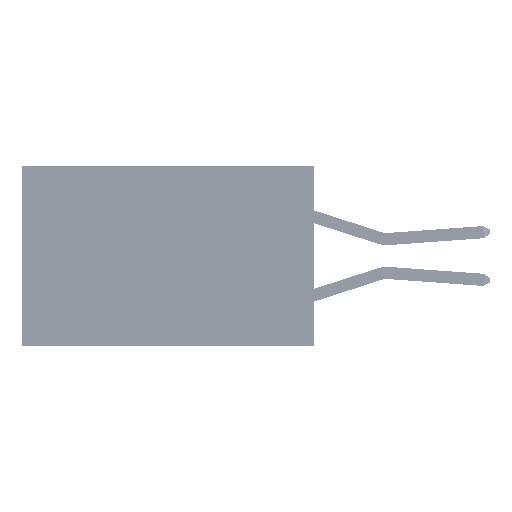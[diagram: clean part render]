
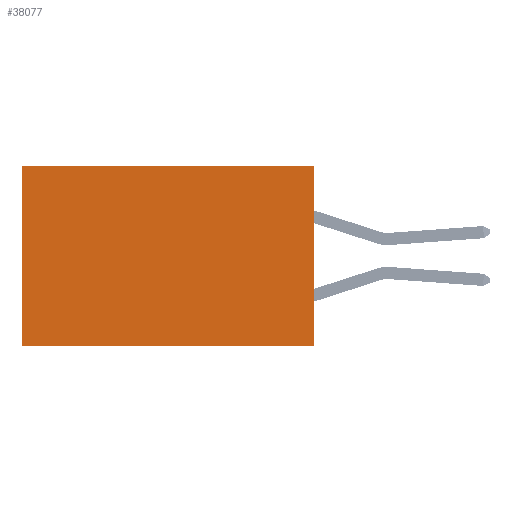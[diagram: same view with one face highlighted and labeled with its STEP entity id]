
A CAD part, left-side view. The second image highlights one B-rep face of the part: STEP entity #38077.
In plain terms, the highlighted planar face has unit normal (-1, 0, 0).
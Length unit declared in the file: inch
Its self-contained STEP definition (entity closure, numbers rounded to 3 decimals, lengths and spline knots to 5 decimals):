
#411 = VERTEX_POINT ( 'NONE', #23533 ) ;
#2952 = ORIENTED_EDGE ( 'NONE', *, *, #38654, .F. ) ;
#3434 = FACE_OUTER_BOUND ( 'NONE', #4018, .T. ) ;
#3687 = ORIENTED_EDGE ( 'NONE', *, *, #8347, .T. ) ;
#4018 = EDGE_LOOP ( 'NONE', ( #3687, #27992, #2952, #43859 ) ) ;
#5990 = VECTOR ( 'NONE', #41328, 39.37008 ) ;
#7865 = EDGE_CURVE ( 'NONE', #411, #35068, #50185, .T. ) ;
#8347 = EDGE_CURVE ( 'NONE', #35068, #29276, #51394, .T. ) ;
#9058 = VECTOR ( 'NONE', #41495, 39.37008 ) ;
#15047 = DIRECTION ( 'NONE',  ( 0., 0., -1. ) ) ;
#17683 = CARTESIAN_POINT ( 'NONE',  ( 0.2875, 0., 0. ) ) ;
#18601 = LINE ( 'NONE', #17683, #9058 ) ;
#19159 = PLANE ( 'NONE',  #27684 ) ;
#20217 = LINE ( 'NONE', #48362, #41045 ) ;
#22515 = CARTESIAN_POINT ( 'NONE',  ( 0.2875, 0., 0. ) ) ;
#23533 = CARTESIAN_POINT ( 'NONE',  ( 0.2875, 0., 0. ) ) ;
#25495 = EDGE_CURVE ( 'NONE', #47057, #29276, #20217, .T. ) ;
#26878 = DIRECTION ( 'NONE',  ( 0., 0., -1. ) ) ;
#27684 = AXIS2_PLACEMENT_3D ( 'NONE', #22515, #30951, #26878 ) ;
#27992 = ORIENTED_EDGE ( 'NONE', *, *, #25495, .F. ) ;
#29276 = VERTEX_POINT ( 'NONE', #45435 ) ;
#30951 = DIRECTION ( 'NONE',  ( 1., 0., 0. ) ) ;
#34372 = CARTESIAN_POINT ( 'NONE',  ( 0.2875, 0., -0.37 ) ) ;
#35068 = VERTEX_POINT ( 'NONE', #37306 ) ;
#36695 = DIRECTION ( 'NONE',  ( 0., 1., 0. ) ) ;
#37306 = CARTESIAN_POINT ( 'NONE',  ( 0.2875, 0.6, 0. ) ) ;
#38077 = ADVANCED_FACE ( 'NONE', ( #3434 ), #19159, .F. ) ;
#38654 = EDGE_CURVE ( 'NONE', #411, #47057, #18601, .T. ) ;
#39779 = CARTESIAN_POINT ( 'NONE',  ( 0.2875, 0.6, 0. ) ) ;
#40691 = VECTOR ( 'NONE', #15047, 39.37008 ) ;
#41045 = VECTOR ( 'NONE', #36695, 39.37008 ) ;
#41328 = DIRECTION ( 'NONE',  ( 0., 1., 0. ) ) ;
#41495 = DIRECTION ( 'NONE',  ( 0., 0., -1. ) ) ;
#43859 = ORIENTED_EDGE ( 'NONE', *, *, #7865, .T. ) ;
#45435 = CARTESIAN_POINT ( 'NONE',  ( 0.2875, 0.6, -0.37 ) ) ;
#47057 = VERTEX_POINT ( 'NONE', #34372 ) ;
#48362 = CARTESIAN_POINT ( 'NONE',  ( 0.2875, 0., -0.37 ) ) ;
#50185 = LINE ( 'NONE', #51665, #5990 ) ;
#51394 = LINE ( 'NONE', #39779, #40691 ) ;
#51665 = CARTESIAN_POINT ( 'NONE',  ( 0.2875, 0., 0. ) ) ;
